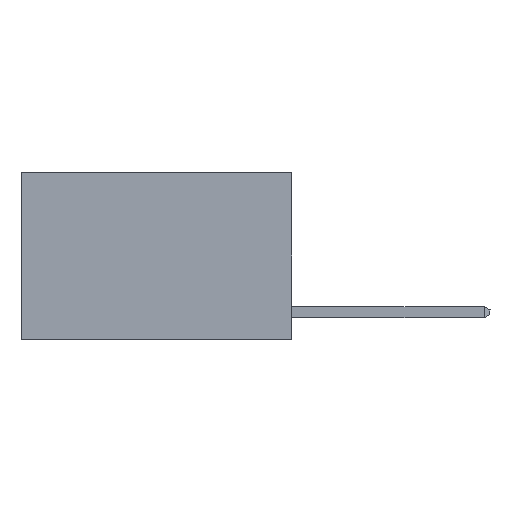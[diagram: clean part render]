
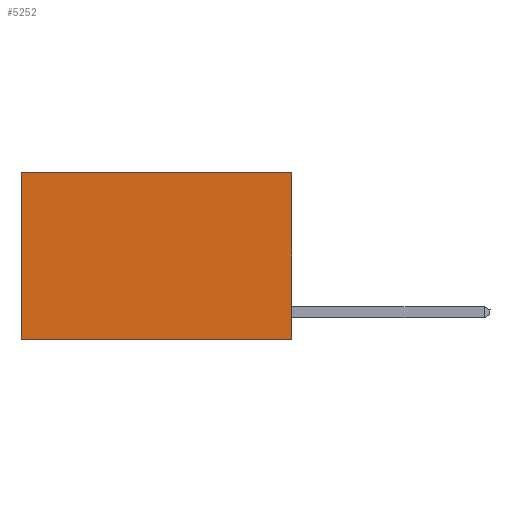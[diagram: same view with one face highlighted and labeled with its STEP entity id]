
A CAD part, left-side view. The second image highlights one B-rep face of the part: STEP entity #5252.
In plain terms, the highlighted planar face has unit normal (-1, 0, 0).
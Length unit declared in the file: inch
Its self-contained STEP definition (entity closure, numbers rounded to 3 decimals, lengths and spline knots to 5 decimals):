
#585 = DIRECTION ( 'NONE',  ( 0., 1., 0. ) ) ;
#844 = FACE_OUTER_BOUND ( 'NONE', #13639, .T. ) ;
#2250 = LINE ( 'NONE', #16554, #19624 ) ;
#3779 = LINE ( 'NONE', #15796, #8401 ) ;
#4228 = LINE ( 'NONE', #21762, #18632 ) ;
#4355 = DIRECTION ( 'NONE',  ( 0., 1., 0. ) ) ;
#5252 = ADVANCED_FACE ( 'NONE', ( #844 ), #19312, .F. ) ;
#5344 = DIRECTION ( 'NONE',  ( 0., 0., -1. ) ) ;
#5769 = ORIENTED_EDGE ( 'NONE', *, *, #8640, .T. ) ;
#7163 = CARTESIAN_POINT ( 'NONE',  ( 0.2625, 0., 0. ) ) ;
#7637 = VERTEX_POINT ( 'NONE', #15213 ) ;
#7944 = CARTESIAN_POINT ( 'NONE',  ( 0.2625, 0., 0. ) ) ;
#7994 = LINE ( 'NONE', #19554, #21249 ) ;
#8401 = VECTOR ( 'NONE', #5344, 39.37008 ) ;
#8640 = EDGE_CURVE ( 'NONE', #19322, #12389, #4228, .T. ) ;
#8910 = DIRECTION ( 'NONE',  ( 1., 0., 0. ) ) ;
#10459 = EDGE_CURVE ( 'NONE', #14343, #19322, #2250, .T. ) ;
#11463 = DIRECTION ( 'NONE',  ( 0., 0., -1. ) ) ;
#12086 = EDGE_CURVE ( 'NONE', #14343, #7637, #3779, .T. ) ;
#12389 = VERTEX_POINT ( 'NONE', #22064 ) ;
#12465 = ORIENTED_EDGE ( 'NONE', *, *, #12086, .F. ) ;
#13639 = EDGE_LOOP ( 'NONE', ( #5769, #19451, #12465, #21647 ) ) ;
#14343 = VERTEX_POINT ( 'NONE', #7944 ) ;
#15213 = CARTESIAN_POINT ( 'NONE',  ( 0.2625, 0., -0.37 ) ) ;
#15796 = CARTESIAN_POINT ( 'NONE',  ( 0.2625, 0., 0. ) ) ;
#15971 = EDGE_CURVE ( 'NONE', #7637, #12389, #7994, .T. ) ;
#16554 = CARTESIAN_POINT ( 'NONE',  ( 0.2625, 0., 0. ) ) ;
#18632 = VECTOR ( 'NONE', #11463, 39.37008 ) ;
#18865 = AXIS2_PLACEMENT_3D ( 'NONE', #7163, #8910, #21023 ) ;
#19312 = PLANE ( 'NONE',  #18865 ) ;
#19322 = VERTEX_POINT ( 'NONE', #21703 ) ;
#19451 = ORIENTED_EDGE ( 'NONE', *, *, #15971, .F. ) ;
#19554 = CARTESIAN_POINT ( 'NONE',  ( 0.2625, 0., -0.37 ) ) ;
#19624 = VECTOR ( 'NONE', #4355, 39.37008 ) ;
#21023 = DIRECTION ( 'NONE',  ( 0., 0., -1. ) ) ;
#21249 = VECTOR ( 'NONE', #585, 39.37008 ) ;
#21647 = ORIENTED_EDGE ( 'NONE', *, *, #10459, .T. ) ;
#21703 = CARTESIAN_POINT ( 'NONE',  ( 0.2625, 0.6, 0. ) ) ;
#21762 = CARTESIAN_POINT ( 'NONE',  ( 0.2625, 0.6, 0. ) ) ;
#22064 = CARTESIAN_POINT ( 'NONE',  ( 0.2625, 0.6, -0.37 ) ) ;
